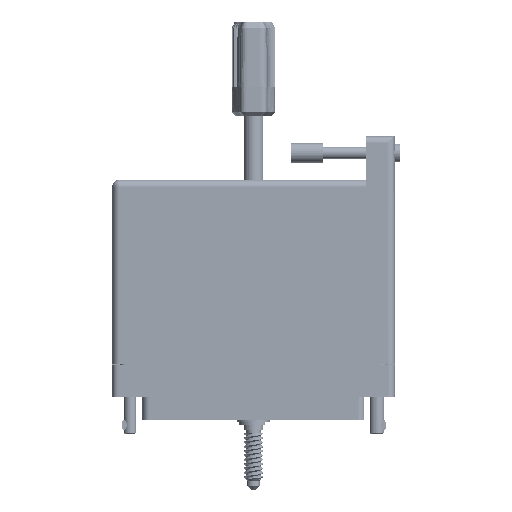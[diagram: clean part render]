
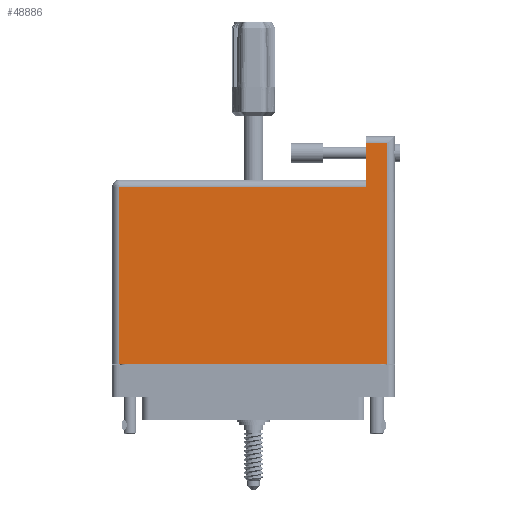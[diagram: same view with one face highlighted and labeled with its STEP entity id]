
A CAD part, front view. The second image highlights one B-rep face of the part: STEP entity #48886.
In plain terms, the highlighted face is planar.
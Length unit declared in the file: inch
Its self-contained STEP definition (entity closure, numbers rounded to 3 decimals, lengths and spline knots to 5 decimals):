
#4689 = EDGE_CURVE ( 'NONE', #43605, #33923, #67207, .T. ) ;
#7185 = CARTESIAN_POINT ( 'NONE',  ( 1.289, 2.095, 0.617 ) ) ;
#8806 = DIRECTION ( 'NONE',  ( 0., 1., 0. ) ) ;
#10666 = DIRECTION ( 'NONE',  ( -1., 0., 0. ) ) ;
#11263 = CARTESIAN_POINT ( 'NONE',  ( -1.289, -0.1, 0.617 ) ) ;
#11905 = DIRECTION ( 'NONE',  ( -1., 0., 0. ) ) ;
#11974 = VECTOR ( 'NONE', #11905, 39.37008 ) ;
#13764 = DIRECTION ( 'NONE',  ( 0., -1., 0. ) ) ;
#13783 = ORIENTED_EDGE ( 'NONE', *, *, #4689, .T. ) ;
#14614 = CARTESIAN_POINT ( 'NONE',  ( 1.079, 2.025, 0.617 ) ) ;
#16220 = CARTESIAN_POINT ( 'NONE',  ( -1.359, -0.1, 0.617 ) ) ;
#16667 = LINE ( 'NONE', #34418, #11974 ) ;
#17256 = FACE_OUTER_BOUND ( 'NONE', #35684, .T. ) ;
#18913 = CARTESIAN_POINT ( 'NONE',  ( -1.359, 1.675, 0.617 ) ) ;
#19941 = LINE ( 'NONE', #16220, #57206 ) ;
#20622 = VECTOR ( 'NONE', #13764, 39.37008 ) ;
#23154 = VECTOR ( 'NONE', #10666, 39.37008 ) ;
#24634 = CARTESIAN_POINT ( 'NONE',  ( 1.289, 2.025, 0.617 ) ) ;
#26442 = LINE ( 'NONE', #7185, #96362 ) ;
#32956 = CARTESIAN_POINT ( 'NONE',  ( 1.079, 2.095, 0.617 ) ) ;
#33923 = VERTEX_POINT ( 'NONE', #11263 ) ;
#34418 = CARTESIAN_POINT ( 'NONE',  ( -1.359, 2.025, 0.617 ) ) ;
#34446 = EDGE_CURVE ( 'NONE', #33923, #62535, #19941, .T. ) ;
#35684 = EDGE_LOOP ( 'NONE', ( #44105, #13783, #93217, #47540, #43534, #47391 ) ) ;
#36580 = EDGE_CURVE ( 'NONE', #56061, #43605, #86050, .T. ) ;
#38203 = LINE ( 'NONE', #32956, #85947 ) ;
#39902 = VERTEX_POINT ( 'NONE', #24634 ) ;
#43534 = ORIENTED_EDGE ( 'NONE', *, *, #70968, .T. ) ;
#43605 = VERTEX_POINT ( 'NONE', #91202 ) ;
#44105 = ORIENTED_EDGE ( 'NONE', *, *, #36580, .T. ) ;
#45356 = EDGE_CURVE ( 'NONE', #62535, #39902, #26442, .T. ) ;
#47360 = VERTEX_POINT ( 'NONE', #14614 ) ;
#47391 = ORIENTED_EDGE ( 'NONE', *, *, #65368, .T. ) ;
#47480 = DIRECTION ( 'NONE',  ( 1., 0., 0. ) ) ;
#47540 = ORIENTED_EDGE ( 'NONE', *, *, #45356, .T. ) ;
#48886 = ADVANCED_FACE ( 'NONE', ( #17256 ), #53749, .F. ) ;
#53749 = PLANE ( 'NONE',  #77300 ) ;
#55288 = CARTESIAN_POINT ( 'NONE',  ( -1.359, 1.605, 0.617 ) ) ;
#56061 = VERTEX_POINT ( 'NONE', #72347 ) ;
#56315 = DIRECTION ( 'NONE',  ( 0., 0., -1. ) ) ;
#57206 = VECTOR ( 'NONE', #47480, 39.37008 ) ;
#62535 = VERTEX_POINT ( 'NONE', #75349 ) ;
#65368 = EDGE_CURVE ( 'NONE', #47360, #56061, #38203, .T. ) ;
#67207 = LINE ( 'NONE', #94967, #20622 ) ;
#70968 = EDGE_CURVE ( 'NONE', #39902, #47360, #16667, .T. ) ;
#72347 = CARTESIAN_POINT ( 'NONE',  ( 1.079, 1.605, 0.617 ) ) ;
#75349 = CARTESIAN_POINT ( 'NONE',  ( 1.289, -0.1, 0.617 ) ) ;
#76829 = DIRECTION ( 'NONE',  ( 0., -1., 0. ) ) ;
#77300 = AXIS2_PLACEMENT_3D ( 'NONE', #18913, #56315, #86306 ) ;
#85947 = VECTOR ( 'NONE', #76829, 39.37008 ) ;
#86050 = LINE ( 'NONE', #55288, #23154 ) ;
#86306 = DIRECTION ( 'NONE',  ( -1., 0., 0. ) ) ;
#91202 = CARTESIAN_POINT ( 'NONE',  ( -1.289, 1.605, 0.617 ) ) ;
#93217 = ORIENTED_EDGE ( 'NONE', *, *, #34446, .T. ) ;
#94967 = CARTESIAN_POINT ( 'NONE',  ( -1.289, -0.1, 0.617 ) ) ;
#96362 = VECTOR ( 'NONE', #8806, 39.37008 ) ;
